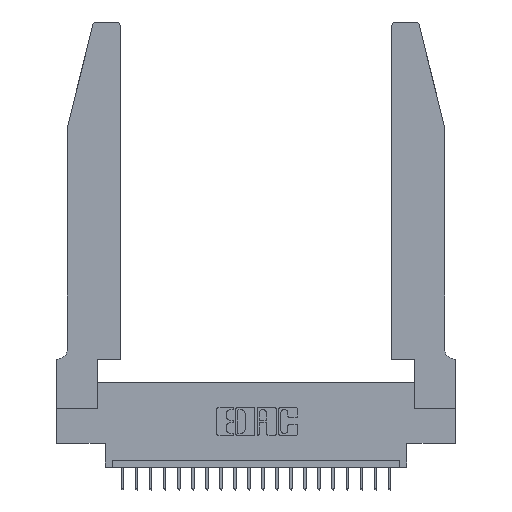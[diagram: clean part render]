
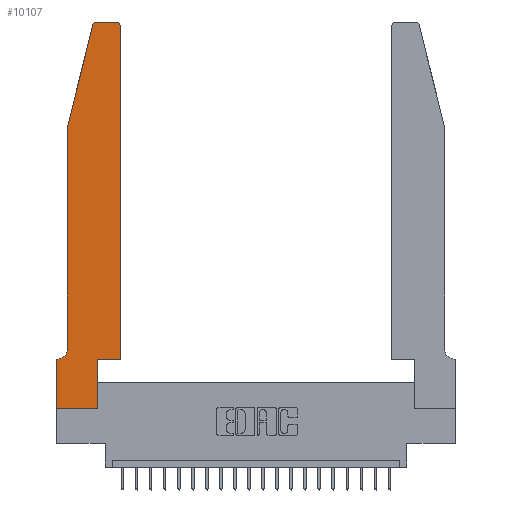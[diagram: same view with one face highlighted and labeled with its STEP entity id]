
A CAD part, top view. The second image highlights one B-rep face of the part: STEP entity #10107.
In plain terms, the highlighted planar face has unit normal (0, 0, 1).
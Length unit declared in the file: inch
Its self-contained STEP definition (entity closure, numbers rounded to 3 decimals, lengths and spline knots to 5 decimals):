
#147 = EDGE_CURVE ( 'NONE', #4366, #13114, #8601, .T. ) ;
#347 = CARTESIAN_POINT ( 'NONE',  ( 0.0755, 0.42, 0.37 ) ) ;
#592 = AXIS2_PLACEMENT_3D ( 'NONE', #3495, #10633, #2213 ) ;
#613 = LINE ( 'NONE', #19997, #9535 ) ;
#801 = VECTOR ( 'NONE', #4872, 39.37008 ) ;
#1008 = VERTEX_POINT ( 'NONE', #17484 ) ;
#1319 = CARTESIAN_POINT ( 'NONE',  ( 0.0755, 2., 0.37 ) ) ;
#1455 = EDGE_CURVE ( 'NONE', #2574, #7156, #18520, .T. ) ;
#1511 = DIRECTION ( 'NONE',  ( 1., 0., 0. ) ) ;
#1713 = ORIENTED_EDGE ( 'NONE', *, *, #19864, .T. ) ;
#1783 = DIRECTION ( 'NONE',  ( 0., -1., 0. ) ) ;
#1933 = EDGE_CURVE ( 'NONE', #10683, #13393, #16274, .T. ) ;
#2213 = DIRECTION ( 'NONE',  ( -1., 0., 0. ) ) ;
#2266 = DIRECTION ( 'NONE',  ( 0., 0., 1. ) ) ;
#2345 = PLANE ( 'NONE',  #7573 ) ;
#2574 = VERTEX_POINT ( 'NONE', #10225 ) ;
#2619 = ORIENTED_EDGE ( 'NONE', *, *, #14502, .T. ) ;
#3216 = CARTESIAN_POINT ( 'NONE',  ( 0.284, 2.75, 0.37 ) ) ;
#3473 = LINE ( 'NONE', #13245, #14873 ) ;
#3495 = CARTESIAN_POINT ( 'NONE',  ( 0.0055, 0.42, 0.37 ) ) ;
#3514 = EDGE_CURVE ( 'NONE', #7156, #1008, #16419, .T. ) ;
#3764 = CARTESIAN_POINT ( 'NONE',  ( 0., 0.35, 0.37 ) ) ;
#4284 = VECTOR ( 'NONE', #18099, 39.37008 ) ;
#4366 = VERTEX_POINT ( 'NONE', #22050 ) ;
#4724 = DIRECTION ( 'NONE',  ( 1., 0., 0. ) ) ;
#4872 = DIRECTION ( 'NONE',  ( 1., 0., 0. ) ) ;
#4882 = DIRECTION ( 'NONE',  ( 0., 0., 1. ) ) ;
#4927 = EDGE_LOOP ( 'NONE', ( #7428, #17126, #15197, #2619, #10262, #1713, #22378, #5031, #17783, #12206, #17019, #19423 ) ) ;
#5031 = ORIENTED_EDGE ( 'NONE', *, *, #147, .T. ) ;
#5448 = EDGE_CURVE ( 'NONE', #17884, #20372, #11360, .T. ) ;
#6059 = CARTESIAN_POINT ( 'NONE',  ( 0., 0.35, 0.37 ) ) ;
#6329 = AXIS2_PLACEMENT_3D ( 'NONE', #13861, #12171, #1511 ) ;
#6383 = DIRECTION ( 'NONE',  ( 1., 0., 0. ) ) ;
#6740 = CARTESIAN_POINT ( 'NONE',  ( 0.2865, 0., 0.37 ) ) ;
#6776 = FACE_OUTER_BOUND ( 'NONE', #4927, .T. ) ;
#7125 = CARTESIAN_POINT ( 'NONE',  ( 0.0755, 2., 0.37 ) ) ;
#7156 = VERTEX_POINT ( 'NONE', #12305 ) ;
#7302 = CARTESIAN_POINT ( 'NONE',  ( 0.2865, 0.35, 0.37 ) ) ;
#7428 = ORIENTED_EDGE ( 'NONE', *, *, #15136, .T. ) ;
#7573 = AXIS2_PLACEMENT_3D ( 'NONE', #6059, #2266, #18550 ) ;
#7973 = LINE ( 'NONE', #21640, #8263 ) ;
#8263 = VECTOR ( 'NONE', #10946, 39.37008 ) ;
#8578 = EDGE_CURVE ( 'NONE', #13114, #11583, #8732, .T. ) ;
#8601 = LINE ( 'NONE', #19720, #801 ) ;
#8631 = CARTESIAN_POINT ( 'NONE',  ( 0.4505, 0.35, 0.37 ) ) ;
#8732 = LINE ( 'NONE', #7302, #4284 ) ;
#9376 = LINE ( 'NONE', #1319, #14405 ) ;
#9535 = VECTOR ( 'NONE', #12979, 39.37008 ) ;
#9977 = VECTOR ( 'NONE', #20002, 39.37008 ) ;
#10107 = ADVANCED_FACE ( 'NONE', ( #6776 ), #2345, .T. ) ;
#10225 = CARTESIAN_POINT ( 'NONE',  ( 0.4505, 0.35, 0.37 ) ) ;
#10245 = LINE ( 'NONE', #16690, #9977 ) ;
#10262 = ORIENTED_EDGE ( 'NONE', *, *, #1933, .T. ) ;
#10633 = DIRECTION ( 'NONE',  ( 0., 0., -1. ) ) ;
#10683 = VERTEX_POINT ( 'NONE', #347 ) ;
#10703 = EDGE_CURVE ( 'NONE', #20372, #17014, #613, .T. ) ;
#10946 = DIRECTION ( 'NONE',  ( -1., 0., 0. ) ) ;
#11180 = CARTESIAN_POINT ( 'NONE',  ( 0.25487, 2.72718, 0.37 ) ) ;
#11360 = CIRCLE ( 'NONE', #6329, 0.03 ) ;
#11583 = VERTEX_POINT ( 'NONE', #15051 ) ;
#12171 = DIRECTION ( 'NONE',  ( 0., 0., 1. ) ) ;
#12206 = ORIENTED_EDGE ( 'NONE', *, *, #16732, .T. ) ;
#12305 = CARTESIAN_POINT ( 'NONE',  ( 0.4505, 2.72, 0.37 ) ) ;
#12979 = DIRECTION ( 'NONE',  ( -0.239, -0.971, 0. ) ) ;
#13114 = VERTEX_POINT ( 'NONE', #6740 ) ;
#13245 = CARTESIAN_POINT ( 'NONE',  ( 0.0755, 0.35, 0.37 ) ) ;
#13393 = VERTEX_POINT ( 'NONE', #17157 ) ;
#13861 = CARTESIAN_POINT ( 'NONE',  ( 0.284, 2.72, 0.37 ) ) ;
#14405 = VECTOR ( 'NONE', #1783, 39.37008 ) ;
#14502 = EDGE_CURVE ( 'NONE', #17014, #10683, #9376, .T. ) ;
#14873 = VECTOR ( 'NONE', #17149, 39.37008 ) ;
#15038 = VECTOR ( 'NONE', #6383, 39.37008 ) ;
#15051 = CARTESIAN_POINT ( 'NONE',  ( 0.2865, 0.35, 0.37 ) ) ;
#15136 = EDGE_CURVE ( 'NONE', #1008, #17884, #7973, .T. ) ;
#15190 = CARTESIAN_POINT ( 'NONE',  ( 0.4505, 0.35, 0.37 ) ) ;
#15197 = ORIENTED_EDGE ( 'NONE', *, *, #10703, .T. ) ;
#16124 = AXIS2_PLACEMENT_3D ( 'NONE', #20743, #4882, #4724 ) ;
#16274 = CIRCLE ( 'NONE', #592, 0.07 ) ;
#16419 = CIRCLE ( 'NONE', #16124, 0.03 ) ;
#16583 = VECTOR ( 'NONE', #18139, 39.37008 ) ;
#16690 = CARTESIAN_POINT ( 'NONE',  ( 0., 0., 0.37 ) ) ;
#16732 = EDGE_CURVE ( 'NONE', #11583, #2574, #21866, .T. ) ;
#17014 = VERTEX_POINT ( 'NONE', #7125 ) ;
#17019 = ORIENTED_EDGE ( 'NONE', *, *, #1455, .T. ) ;
#17126 = ORIENTED_EDGE ( 'NONE', *, *, #5448, .T. ) ;
#17149 = DIRECTION ( 'NONE',  ( -1., 0., 0. ) ) ;
#17157 = CARTESIAN_POINT ( 'NONE',  ( 0.0055, 0.35, 0.37 ) ) ;
#17169 = EDGE_CURVE ( 'NONE', #20825, #4366, #10245, .T. ) ;
#17484 = CARTESIAN_POINT ( 'NONE',  ( 0.4205, 2.75, 0.37 ) ) ;
#17783 = ORIENTED_EDGE ( 'NONE', *, *, #8578, .T. ) ;
#17884 = VERTEX_POINT ( 'NONE', #3216 ) ;
#18099 = DIRECTION ( 'NONE',  ( 0., 1., 0. ) ) ;
#18139 = DIRECTION ( 'NONE',  ( 0., 1., 0. ) ) ;
#18520 = LINE ( 'NONE', #8631, #16583 ) ;
#18550 = DIRECTION ( 'NONE',  ( 1., 0., 0. ) ) ;
#19423 = ORIENTED_EDGE ( 'NONE', *, *, #3514, .T. ) ;
#19720 = CARTESIAN_POINT ( 'NONE',  ( 0., 0., 0.37 ) ) ;
#19864 = EDGE_CURVE ( 'NONE', #13393, #20825, #3473, .T. ) ;
#19997 = CARTESIAN_POINT ( 'NONE',  ( 0.0755, 2., 0.37 ) ) ;
#20002 = DIRECTION ( 'NONE',  ( 0., -1., 0. ) ) ;
#20372 = VERTEX_POINT ( 'NONE', #11180 ) ;
#20743 = CARTESIAN_POINT ( 'NONE',  ( 0.4205, 2.72, 0.37 ) ) ;
#20825 = VERTEX_POINT ( 'NONE', #3764 ) ;
#21640 = CARTESIAN_POINT ( 'NONE',  ( 0.2605, 2.75, 0.37 ) ) ;
#21866 = LINE ( 'NONE', #15190, #15038 ) ;
#22050 = CARTESIAN_POINT ( 'NONE',  ( 0., 0., 0.37 ) ) ;
#22378 = ORIENTED_EDGE ( 'NONE', *, *, #17169, .T. ) ;
